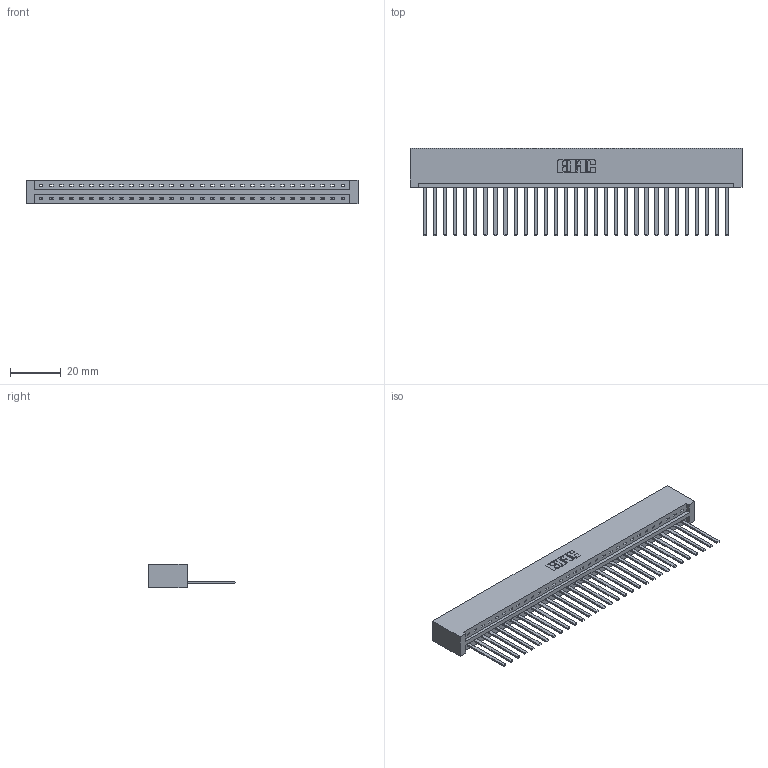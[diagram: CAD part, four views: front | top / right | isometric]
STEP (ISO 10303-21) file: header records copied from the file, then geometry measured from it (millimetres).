
FILE_DESCRIPTION (( 'STEP AP203' ), '1' );
FILE_NAME ('387-031-544-101.STEP', '2018-09-18T04:56:04', ( '' ), ( '' ), 'SwSTEP 2.0', 'SolidWorks 2016', '' );
FILE_SCHEMA (( 'CONFIG_CONTROL_DESIGN' ));
Length unit declared in the file: inch
Products named in the file (3): 345-292-001_345-293-144; 387-031-544-101; 337 Part_No Mounting Lugs
Assembly tree (32 placements, depth 2):
  387-031-544-101
    337 Part_No Mounting Lugs
    345-292-001_345-293-144  x31
Bounding box: 130.71 x 34.3 x 9.4 mm (x, y, z)
Volume: 14545 mm3; surface area: 16131.5 mm2
Topology: 32 solids, 32 shells, 1842 faces, 5557 edges, 3662 vertices
Faces by surface type: plane 1368, cylinder 474
Entity records: 24005 total; most frequent: CARTESIAN_POINT 4187, ORIENTED_EDGE 4154, DIRECTION 3535, EDGE_CURVE 2077, LINE 1961, VECTOR 1961, VERTEX_POINT 1382, AXIS2_PLACEMENT_3D 787
